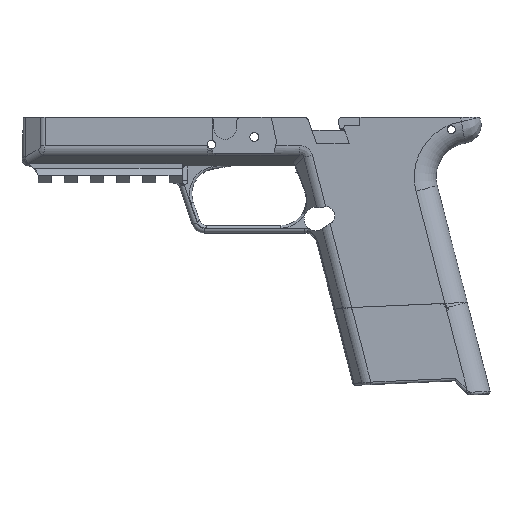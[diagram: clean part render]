
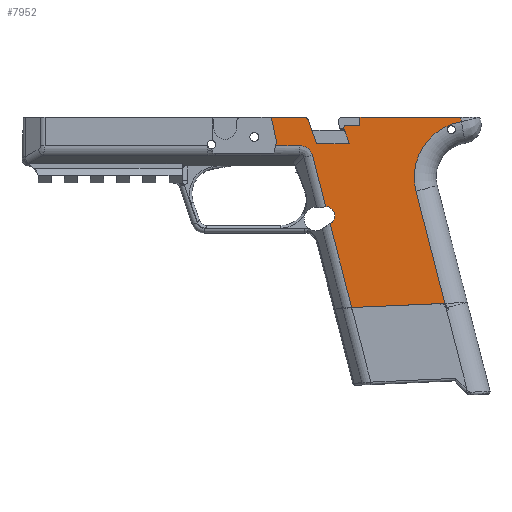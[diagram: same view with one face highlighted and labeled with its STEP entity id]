
A CAD part, left-side view. The second image highlights one B-rep face of the part: STEP entity #7952.
In plain terms, the highlighted face is planar.
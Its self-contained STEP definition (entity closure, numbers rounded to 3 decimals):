
#211=CIRCLE('',#8522,1.);
#212=CIRCLE('',#8524,2.);
#213=CIRCLE('',#8526,3.585);
#214=CIRCLE('',#8527,2.921);
#215=CIRCLE('',#8528,3.585);
#216=CIRCLE('',#8529,22.475);
#217=CIRCLE('',#8530,7.5);
#659=FACE_OUTER_BOUND('',#1107,.T.);
#1107=EDGE_LOOP('',(#5929,#5930,#5931,#5932,#5933,#5934,#5935,#5936,#5937,
#5938,#5939,#5940,#5941,#5942,#5943,#5944,#5945,#5946,#5947,#5948,#5949,
#5950,#5951));
#1680=LINE('',#13138,#2407);
#1681=LINE('',#13140,#2408);
#1682=LINE('',#13142,#2409);
#1683=LINE('',#13146,#2410);
#1684=LINE('',#13148,#2411);
#1685=LINE('',#13150,#2412);
#1686=LINE('',#13152,#2413);
#1687=LINE('',#13156,#2414);
#1688=LINE('',#13164,#2415);
#1689=LINE('',#13166,#2416);
#1690=LINE('',#13168,#2417);
#1691=LINE('',#13170,#2418);
#1692=LINE('',#13176,#2419);
#1693=LINE('',#13178,#2420);
#1694=LINE('',#13179,#2421);
#2407=VECTOR('',#9794,10.);
#2408=VECTOR('',#9795,10.);
#2409=VECTOR('',#9796,10.);
#2410=VECTOR('',#9799,10.);
#2411=VECTOR('',#9800,10.);
#2412=VECTOR('',#9801,10.);
#2413=VECTOR('',#9802,10.);
#2414=VECTOR('',#9805,10.);
#2415=VECTOR('',#9812,10.);
#2416=VECTOR('',#9813,10.);
#2417=VECTOR('',#9814,10.);
#2418=VECTOR('',#9815,10.);
#2419=VECTOR('',#9820,10.);
#2420=VECTOR('',#9821,10.);
#2421=VECTOR('',#9822,10.);
#2918=ELLIPSE('',#8525,10.693,7.);
#3439=VERTEX_POINT('',#13131);
#3440=VERTEX_POINT('',#13133);
#3441=VERTEX_POINT('',#13137);
#3442=VERTEX_POINT('',#13139);
#3443=VERTEX_POINT('',#13141);
#3444=VERTEX_POINT('',#13143);
#3445=VERTEX_POINT('',#13145);
#3446=VERTEX_POINT('',#13147);
#3447=VERTEX_POINT('',#13149);
#3448=VERTEX_POINT('',#13151);
#3449=VERTEX_POINT('',#13153);
#3450=VERTEX_POINT('',#13155);
#3451=VERTEX_POINT('',#13157);
#3452=VERTEX_POINT('',#13159);
#3453=VERTEX_POINT('',#13161);
#3454=VERTEX_POINT('',#13163);
#3455=VERTEX_POINT('',#13165);
#3456=VERTEX_POINT('',#13167);
#3457=VERTEX_POINT('',#13169);
#3458=VERTEX_POINT('',#13171);
#3459=VERTEX_POINT('',#13173);
#3460=VERTEX_POINT('',#13175);
#3461=VERTEX_POINT('',#13177);
#4356=EDGE_CURVE('',#3439,#3440,#211,.T.);
#4358=EDGE_CURVE('',#3439,#3441,#1680,.F.);
#4359=EDGE_CURVE('',#3441,#3442,#1681,.T.);
#4360=EDGE_CURVE('',#3442,#3443,#1682,.F.);
#4361=EDGE_CURVE('',#3444,#3443,#212,.T.);
#4362=EDGE_CURVE('',#3444,#3445,#1683,.T.);
#4363=EDGE_CURVE('',#3445,#3446,#1684,.T.);
#4364=EDGE_CURVE('',#3446,#3447,#1685,.T.);
#4365=EDGE_CURVE('',#3448,#3447,#1686,.T.);
#4366=EDGE_CURVE('',#3449,#3448,#2918,.T.);
#4367=EDGE_CURVE('',#3450,#3449,#1687,.T.);
#4368=EDGE_CURVE('',#3450,#3451,#213,.T.);
#4369=EDGE_CURVE('',#3451,#3452,#214,.T.);
#4370=EDGE_CURVE('',#3452,#3453,#215,.T.);
#4371=EDGE_CURVE('',#3453,#3454,#1688,.T.);
#4372=EDGE_CURVE('',#3455,#3454,#1689,.T.);
#4373=EDGE_CURVE('',#3456,#3455,#1690,.T.);
#4374=EDGE_CURVE('',#3457,#3456,#1691,.T.);
#4375=EDGE_CURVE('',#3458,#3457,#216,.T.);
#4376=EDGE_CURVE('',#3459,#3458,#217,.T.);
#4377=EDGE_CURVE('',#3459,#3460,#1692,.T.);
#4378=EDGE_CURVE('',#3460,#3461,#1693,.F.);
#4379=EDGE_CURVE('',#3461,#3440,#1694,.T.);
#5929=ORIENTED_EDGE('',*,*,#4356,.F.);
#5930=ORIENTED_EDGE('',*,*,#4358,.T.);
#5931=ORIENTED_EDGE('',*,*,#4359,.T.);
#5932=ORIENTED_EDGE('',*,*,#4360,.T.);
#5933=ORIENTED_EDGE('',*,*,#4361,.F.);
#5934=ORIENTED_EDGE('',*,*,#4362,.T.);
#5935=ORIENTED_EDGE('',*,*,#4363,.T.);
#5936=ORIENTED_EDGE('',*,*,#4364,.T.);
#5937=ORIENTED_EDGE('',*,*,#4365,.F.);
#5938=ORIENTED_EDGE('',*,*,#4366,.F.);
#5939=ORIENTED_EDGE('',*,*,#4367,.F.);
#5940=ORIENTED_EDGE('',*,*,#4368,.T.);
#5941=ORIENTED_EDGE('',*,*,#4369,.T.);
#5942=ORIENTED_EDGE('',*,*,#4370,.T.);
#5943=ORIENTED_EDGE('',*,*,#4371,.T.);
#5944=ORIENTED_EDGE('',*,*,#4372,.F.);
#5945=ORIENTED_EDGE('',*,*,#4373,.F.);
#5946=ORIENTED_EDGE('',*,*,#4374,.F.);
#5947=ORIENTED_EDGE('',*,*,#4375,.F.);
#5948=ORIENTED_EDGE('',*,*,#4376,.F.);
#5949=ORIENTED_EDGE('',*,*,#4377,.T.);
#5950=ORIENTED_EDGE('',*,*,#4378,.T.);
#5951=ORIENTED_EDGE('',*,*,#4379,.T.);
#7664=PLANE('',#8523);
#7952=ADVANCED_FACE('',(#659),#7664,.F.);
#8522=AXIS2_PLACEMENT_3D('',#13134,#9789,#9790);
#8523=AXIS2_PLACEMENT_3D('',#13136,#9792,#9793);
#8524=AXIS2_PLACEMENT_3D('',#13144,#9797,#9798);
#8525=AXIS2_PLACEMENT_3D('',#13154,#9803,#9804);
#8526=AXIS2_PLACEMENT_3D('',#13158,#9806,#9807);
#8527=AXIS2_PLACEMENT_3D('',#13160,#9808,#9809);
#8528=AXIS2_PLACEMENT_3D('',#13162,#9810,#9811);
#8529=AXIS2_PLACEMENT_3D('',#13172,#9816,#9817);
#8530=AXIS2_PLACEMENT_3D('',#13174,#9818,#9819);
#9789=DIRECTION('center_axis',(-1.,0.,0.));
#9790=DIRECTION('ref_axis',(0.,0.817,-0.576));
#9792=DIRECTION('center_axis',(-1.,0.,0.));
#9793=DIRECTION('ref_axis',(0.,1.,0.));
#9794=DIRECTION('',(0.,0.336,-0.942));
#9795=DIRECTION('',(0.,1.,0.));
#9796=DIRECTION('',(0.,-0.336,0.942));
#9797=DIRECTION('center_axis',(-1.,0.,0.));
#9798=DIRECTION('ref_axis',(0.,-0.576,-0.817));
#9799=DIRECTION('',(0.,1.,0.));
#9800=DIRECTION('',(0.,-0.21,0.978));
#9801=DIRECTION('',(0.,0.21,0.978));
#9802=DIRECTION('',(0.,1.,0.));
#9803=DIRECTION('center_axis',(1.,0.,0.));
#9804=DIRECTION('ref_axis',(0.,-0.714,-0.7));
#9805=DIRECTION('',(0.,0.249,-0.969));
#9806=DIRECTION('center_axis',(-1.,0.,0.));
#9807=DIRECTION('ref_axis',(0.,1.,0.));
#9808=DIRECTION('center_axis',(-1.,0.,0.));
#9809=DIRECTION('ref_axis',(0.,1.,0.));
#9810=DIRECTION('center_axis',(-1.,0.,0.));
#9811=DIRECTION('ref_axis',(0.,1.,0.));
#9812=DIRECTION('',(0.,0.828,0.56));
#9813=DIRECTION('',(0.,0.249,-0.969));
#9814=DIRECTION('',(0.,0.999,0.044));
#9815=DIRECTION('',(0.,-0.249,0.969));
#9816=DIRECTION('center_axis',(1.,0.,0.));
#9817=DIRECTION('ref_axis',(0.,0.,1.));
#9818=DIRECTION('center_axis',(1.,0.,0.));
#9819=DIRECTION('ref_axis',(0.,-0.97,-0.244));
#9820=DIRECTION('',(0.,1.,0.));
#9821=DIRECTION('',(0.,0.,-1.));
#9822=DIRECTION('',(0.,1.,0.));
#13131=CARTESIAN_POINT('',(22.175,-34.374,-2.995));
#13133=CARTESIAN_POINT('',(22.175,-35.316,-4.331));
#13134=CARTESIAN_POINT('Origin',(22.175,-35.316,-3.331));
#13136=CARTESIAN_POINT('Origin',(22.175,-7.921,2.186));
#13137=CARTESIAN_POINT('',(22.175,-36.514,3.));
#13138=CARTESIAN_POINT('',(22.175,-32.976,-6.913));
#13139=CARTESIAN_POINT('',(22.175,-23.407,3.));
#13140=CARTESIAN_POINT('',(22.175,-23.764,3.));
#13141=CARTESIAN_POINT('',(22.175,-20.114,-6.228));
#13142=CARTESIAN_POINT('',(22.175,-21.552,-2.199));
#13143=CARTESIAN_POINT('',(22.175,-18.23,-7.556));
#13144=CARTESIAN_POINT('Origin',(22.175,-18.23,-5.556));
#13145=CARTESIAN_POINT('',(22.175,-5.3,-7.556));
#13146=CARTESIAN_POINT('',(22.175,-86.951,-7.556));
#13147=CARTESIAN_POINT('',(22.175,-7.389,2.186));
#13148=CARTESIAN_POINT('',(22.175,-6.356,-2.63));
#13149=CARTESIAN_POINT('',(22.175,-7.025,3.884));
#13150=CARTESIAN_POINT('',(22.175,-7.4,2.132));
#13151=CARTESIAN_POINT('',(22.175,-16.536,3.884));
#13152=CARTESIAN_POINT('',(22.175,33.814,3.884));
#13153=CARTESIAN_POINT('',(22.175,-21.783,7.651));
#13154=CARTESIAN_POINT('Origin',(22.175,-12.907,12.884));
#13155=CARTESIAN_POINT('',(22.175,-27.074,28.233));
#13156=CARTESIAN_POINT('',(22.175,-26.659,26.619));
#13157=CARTESIAN_POINT('',(22.175,-30.502,30.561));
#13158=CARTESIAN_POINT('Origin',(22.175,-27.144,31.817));
#13159=CARTESIAN_POINT('',(22.175,-30.617,30.925));
#13160=CARTESIAN_POINT('Origin',(22.175,-27.779,31.618));
#13161=CARTESIAN_POINT('',(22.175,-29.153,34.787));
#13162=CARTESIAN_POINT('Origin',(22.175,-27.144,31.817));
#13163=CARTESIAN_POINT('',(22.175,-28.817,35.014));
#13164=CARTESIAN_POINT('',(22.175,-27.054,36.207));
#13165=CARTESIAN_POINT('',(22.175,-37.447,68.587));
#13166=CARTESIAN_POINT('',(22.175,-26.659,26.619));
#13167=CARTESIAN_POINT('',(22.175,-74.722,66.935));
#13168=CARTESIAN_POINT('',(22.175,-40.785,68.439));
#13169=CARTESIAN_POINT('',(22.175,-63.184,22.049));
#13170=CARTESIAN_POINT('',(22.175,-75.103,68.418));
#13171=CARTESIAN_POINT('',(22.175,-81.332,-5.728));
#13172=CARTESIAN_POINT('Origin',(22.175,-84.951,16.453));
#13173=CARTESIAN_POINT('',(22.175,-81.106,-7.556));
#13174=CARTESIAN_POINT('Origin',(22.175,-88.606,-7.556));
#13175=CARTESIAN_POINT('',(22.175,-40.774,-7.556));
#13176=CARTESIAN_POINT('',(22.175,-84.951,-7.556));
#13177=CARTESIAN_POINT('',(22.175,-40.774,-4.331));
#13178=CARTESIAN_POINT('',(22.175,-40.774,-2.685));
#13179=CARTESIAN_POINT('',(22.175,-20.598,-4.331));
